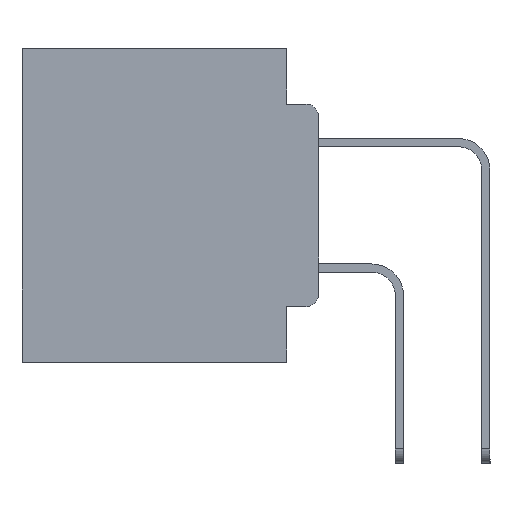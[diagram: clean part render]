
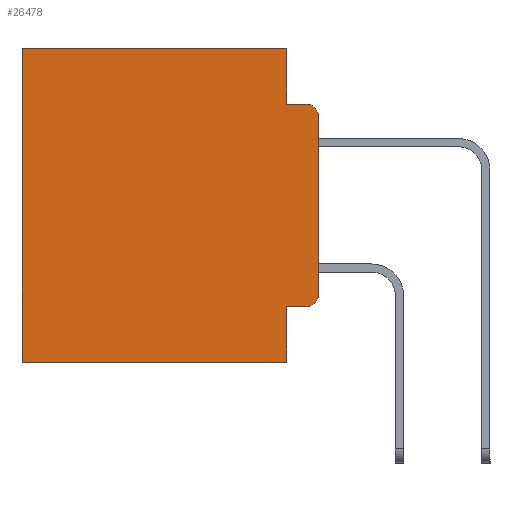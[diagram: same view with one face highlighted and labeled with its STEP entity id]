
A CAD part, left-side view. The second image highlights one B-rep face of the part: STEP entity #26478.
In plain terms, the highlighted planar face has unit normal (-1, 0, 0).
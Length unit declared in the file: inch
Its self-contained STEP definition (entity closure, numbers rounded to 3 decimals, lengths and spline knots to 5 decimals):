
#301 = ORIENTED_EDGE ( 'NONE', *, *, #21222, .T. ) ;
#415 = ORIENTED_EDGE ( 'NONE', *, *, #968, .T. ) ;
#623 = EDGE_LOOP ( 'NONE', ( #7498, #19014, #15678, #9569, #19630, #301, #26570, #24127, #5576, #415 ) ) ;
#639 = LINE ( 'NONE', #6759, #30048 ) ;
#779 = VERTEX_POINT ( 'NONE', #27113 ) ;
#968 = EDGE_CURVE ( 'NONE', #27517, #26977, #27038, .T. ) ;
#1704 = LINE ( 'NONE', #18675, #13555 ) ;
#2882 = CARTESIAN_POINT ( 'NONE',  ( 0.298, 0., 0. ) ) ;
#2904 = CARTESIAN_POINT ( 'NONE',  ( 0.298, 0.02, -0.3915 ) ) ;
#3266 = DIRECTION ( 'NONE',  ( -1., 0., 0. ) ) ;
#3381 = CARTESIAN_POINT ( 'NONE',  ( 0.298, 0.051, -0.0885 ) ) ;
#3419 = VERTEX_POINT ( 'NONE', #3381 ) ;
#3447 = EDGE_CURVE ( 'NONE', #3419, #17908, #639, .T. ) ;
#3688 = VECTOR ( 'NONE', #6970, 39.37008 ) ;
#4279 = EDGE_CURVE ( 'NONE', #21776, #17908, #16507, .T. ) ;
#4489 = VERTEX_POINT ( 'NONE', #9800 ) ;
#4784 = CARTESIAN_POINT ( 'NONE',  ( 0.298, 0., -0.3915 ) ) ;
#5349 = DIRECTION ( 'NONE',  ( 0., 0., -1. ) ) ;
#5519 = LINE ( 'NONE', #6157, #12512 ) ;
#5576 = ORIENTED_EDGE ( 'NONE', *, *, #6760, .T. ) ;
#5757 = CARTESIAN_POINT ( 'NONE',  ( 0.298, 0., 0. ) ) ;
#6157 = CARTESIAN_POINT ( 'NONE',  ( 0.298, 0., -0.5 ) ) ;
#6353 = VERTEX_POINT ( 'NONE', #13724 ) ;
#6759 = CARTESIAN_POINT ( 'NONE',  ( 0.298, 0.051, -0.0885 ) ) ;
#6760 = EDGE_CURVE ( 'NONE', #779, #27517, #13104, .T. ) ;
#6911 = VECTOR ( 'NONE', #11979, 39.37008 ) ;
#6970 = DIRECTION ( 'NONE',  ( 0., 0., -1. ) ) ;
#7465 = CARTESIAN_POINT ( 'NONE',  ( 0.298, 0.02, -0.0885 ) ) ;
#7498 = ORIENTED_EDGE ( 'NONE', *, *, #26596, .F. ) ;
#8170 = DIRECTION ( 'NONE',  ( 0., 0., -1. ) ) ;
#9569 = ORIENTED_EDGE ( 'NONE', *, *, #27331, .F. ) ;
#9634 = LINE ( 'NONE', #5757, #27169 ) ;
#9800 = CARTESIAN_POINT ( 'NONE',  ( 0.298, 0.473, -0.5 ) ) ;
#10483 = EDGE_CURVE ( 'NONE', #779, #13179, #21541, .T. ) ;
#10544 = AXIS2_PLACEMENT_3D ( 'NONE', #16913, #16710, #16611 ) ;
#11979 = DIRECTION ( 'NONE',  ( 0., -1., 0. ) ) ;
#12512 = VECTOR ( 'NONE', #22306, 39.37008 ) ;
#13104 = LINE ( 'NONE', #13193, #6911 ) ;
#13179 = VERTEX_POINT ( 'NONE', #28991 ) ;
#13193 = CARTESIAN_POINT ( 'NONE',  ( 0.298, 0.051, -0.4115 ) ) ;
#13555 = VECTOR ( 'NONE', #20965, 39.37008 ) ;
#13724 = CARTESIAN_POINT ( 'NONE',  ( 0.298, 0.051, 0. ) ) ;
#14617 = PLANE ( 'NONE',  #29934 ) ;
#14938 = EDGE_CURVE ( 'NONE', #13179, #4489, #5519, .T. ) ;
#15678 = ORIENTED_EDGE ( 'NONE', *, *, #3447, .F. ) ;
#15768 = CARTESIAN_POINT ( 'NONE',  ( 0.298, 0., 0. ) ) ;
#16507 = CIRCLE ( 'NONE', #10544, 0.02 ) ;
#16611 = DIRECTION ( 'NONE',  ( 0., 0., -1. ) ) ;
#16710 = DIRECTION ( 'NONE',  ( -1., 0., 0. ) ) ;
#16913 = CARTESIAN_POINT ( 'NONE',  ( 0.298, 0.02, -0.1085 ) ) ;
#17908 = VERTEX_POINT ( 'NONE', #7465 ) ;
#18107 = DIRECTION ( 'NONE',  ( 0., 1., 0. ) ) ;
#18509 = CARTESIAN_POINT ( 'NONE',  ( 0.298, 0.051, 0. ) ) ;
#18619 = FACE_OUTER_BOUND ( 'NONE', #623, .T. ) ;
#18675 = CARTESIAN_POINT ( 'NONE',  ( 0.298, 0.473, 0. ) ) ;
#19014 = ORIENTED_EDGE ( 'NONE', *, *, #4279, .T. ) ;
#19260 = DIRECTION ( 'NONE',  ( 1., 0., 0. ) ) ;
#19630 = ORIENTED_EDGE ( 'NONE', *, *, #27449, .T. ) ;
#20744 = VECTOR ( 'NONE', #18107, 39.37008 ) ;
#20965 = DIRECTION ( 'NONE',  ( 0., 0., -1. ) ) ;
#21222 = EDGE_CURVE ( 'NONE', #23843, #4489, #1704, .T. ) ;
#21541 = LINE ( 'NONE', #18509, #3688 ) ;
#21776 = VERTEX_POINT ( 'NONE', #23441 ) ;
#22087 = CARTESIAN_POINT ( 'NONE',  ( 0.298, 0.051, 0. ) ) ;
#22306 = DIRECTION ( 'NONE',  ( 0., 1., 0. ) ) ;
#23441 = CARTESIAN_POINT ( 'NONE',  ( 0.298, 0., -0.1085 ) ) ;
#23625 = VECTOR ( 'NONE', #24523, 39.37008 ) ;
#23843 = VERTEX_POINT ( 'NONE', #28083 ) ;
#24127 = ORIENTED_EDGE ( 'NONE', *, *, #10483, .F. ) ;
#24523 = DIRECTION ( 'NONE',  ( 0., 0., -1. ) ) ;
#25116 = CARTESIAN_POINT ( 'NONE',  ( 0.298, 0.02, -0.4115 ) ) ;
#26171 = DIRECTION ( 'NONE',  ( 0., -1., 0. ) ) ;
#26246 = DIRECTION ( 'NONE',  ( 0., 0., -1. ) ) ;
#26478 = ADVANCED_FACE ( 'NONE', ( #18619 ), #14617, .F. ) ;
#26570 = ORIENTED_EDGE ( 'NONE', *, *, #14938, .F. ) ;
#26596 = EDGE_CURVE ( 'NONE', #21776, #26977, #9634, .T. ) ;
#26822 = LINE ( 'NONE', #15768, #20744 ) ;
#26977 = VERTEX_POINT ( 'NONE', #4784 ) ;
#27038 = CIRCLE ( 'NONE', #29041, 0.02 ) ;
#27113 = CARTESIAN_POINT ( 'NONE',  ( 0.298, 0.051, -0.4115 ) ) ;
#27169 = VECTOR ( 'NONE', #8170, 39.37008 ) ;
#27331 = EDGE_CURVE ( 'NONE', #6353, #3419, #29629, .T. ) ;
#27449 = EDGE_CURVE ( 'NONE', #6353, #23843, #26822, .T. ) ;
#27517 = VERTEX_POINT ( 'NONE', #25116 ) ;
#28083 = CARTESIAN_POINT ( 'NONE',  ( 0.298, 0.473, 0. ) ) ;
#28991 = CARTESIAN_POINT ( 'NONE',  ( 0.298, 0.051, -0.5 ) ) ;
#29041 = AXIS2_PLACEMENT_3D ( 'NONE', #2904, #3266, #26246 ) ;
#29629 = LINE ( 'NONE', #22087, #23625 ) ;
#29934 = AXIS2_PLACEMENT_3D ( 'NONE', #2882, #19260, #5349 ) ;
#30048 = VECTOR ( 'NONE', #26171, 39.37008 ) ;
